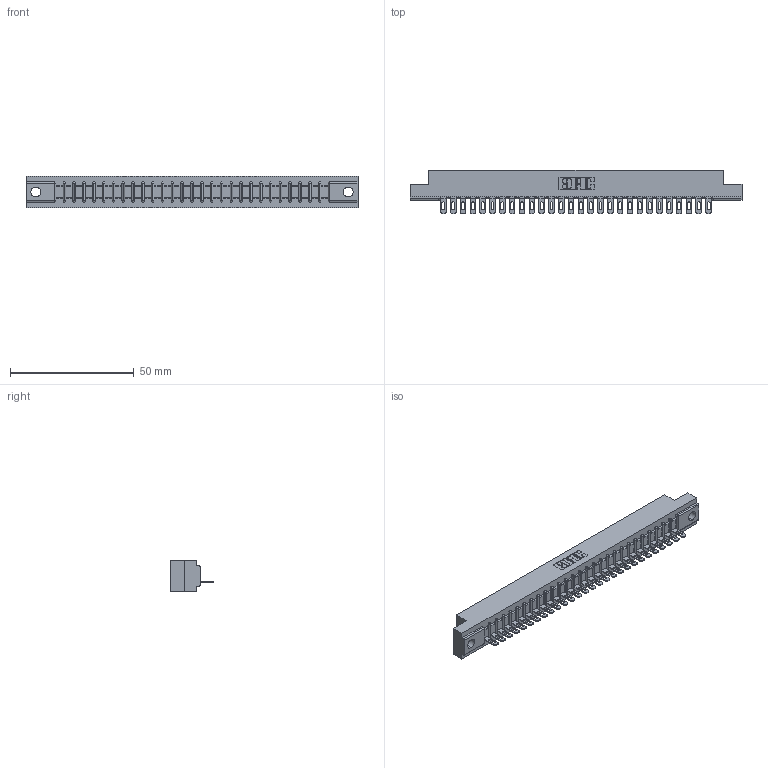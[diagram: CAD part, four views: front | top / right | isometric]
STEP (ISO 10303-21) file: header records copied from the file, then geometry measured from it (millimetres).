
FILE_DESCRIPTION (( 'STEP AP203' ), '1' );
FILE_NAME ('357-028-501-102.STEP', '2018-08-09T05:53:38', ( '' ), ( '' ), 'SwSTEP 2.0', 'SolidWorks 2016', '' );
FILE_SCHEMA (( 'CONFIG_CONTROL_DESIGN' ));
Length unit declared in the file: inch
Products named in the file (3): 307 Part_.128 Dia Mounting Holes; 307-290-002_501; 357-028-501-102
Assembly tree (29 placements, depth 2):
  357-028-501-102
    307 Part_.128 Dia Mounting Holes
    307-290-002_501  x28
Bounding box: 133.96 x 17.42 x 12.7 mm (x, y, z)
Volume: 14167.5 mm3; surface area: 17499.7 mm2
Topology: 29 solids, 29 shells, 2275 faces, 6987 edges, 4578 vertices
Faces by surface type: plane 1302, cylinder 915, sphere 58
Entity records: 26526 total; most frequent: CARTESIAN_POINT 4472, ORIENTED_EDGE 4462, DIRECTION 4355, EDGE_CURVE 2231, LINE 1697, VECTOR 1697, VERTEX_POINT 1446, AXIS2_PLACEMENT_3D 1329
